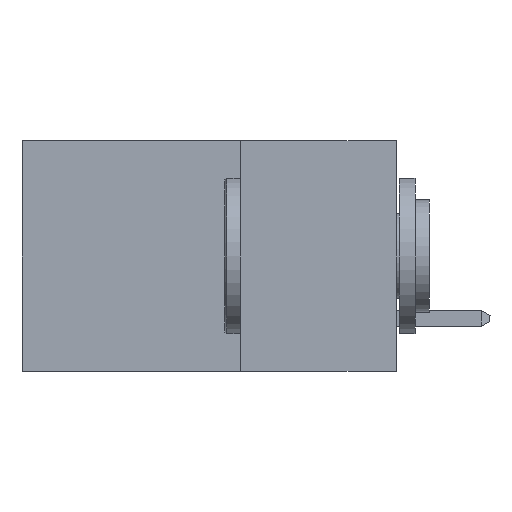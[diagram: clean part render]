
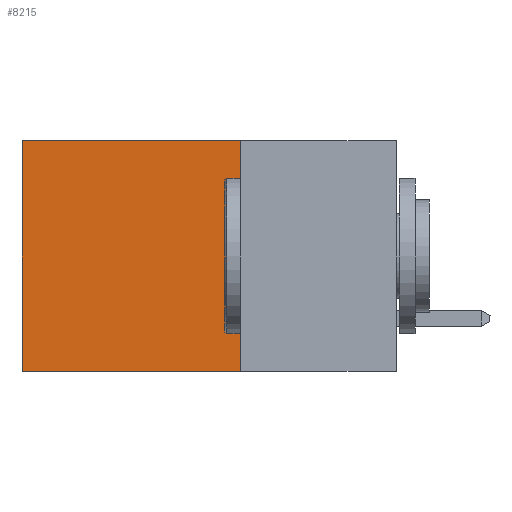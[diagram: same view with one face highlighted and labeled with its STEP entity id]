
A CAD part, left-side view. The second image highlights one B-rep face of the part: STEP entity #8215.
In plain terms, the highlighted planar face has unit normal (-1, 0, 0).
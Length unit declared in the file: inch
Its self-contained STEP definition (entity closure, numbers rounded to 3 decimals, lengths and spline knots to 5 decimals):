
#244 = VECTOR ( 'NONE', #9530, 39.37008 ) ;
#366 = VECTOR ( 'NONE', #10708, 39.37008 ) ;
#685 = VERTEX_POINT ( 'NONE', #2486 ) ;
#753 = EDGE_CURVE ( 'NONE', #7924, #6056, #8800, .T. ) ;
#1277 = EDGE_LOOP ( 'NONE', ( #5672, #1853, #2926, #5214 ) ) ;
#1853 = ORIENTED_EDGE ( 'NONE', *, *, #2600, .F. ) ;
#2177 = CARTESIAN_POINT ( 'NONE',  ( 0.2615, 0.25, -0.37 ) ) ;
#2486 = CARTESIAN_POINT ( 'NONE',  ( 0.2615, 0.6, -0.37 ) ) ;
#2600 = EDGE_CURVE ( 'NONE', #6056, #685, #5330, .T. ) ;
#2926 = ORIENTED_EDGE ( 'NONE', *, *, #753, .F. ) ;
#3370 = CARTESIAN_POINT ( 'NONE',  ( 0.2615, 0.25, -0.37 ) ) ;
#3420 = DIRECTION ( 'NONE',  ( 0., 0., -1. ) ) ;
#4081 = LINE ( 'NONE', #4215, #244 ) ;
#4215 = CARTESIAN_POINT ( 'NONE',  ( 0.2615, 0.6, -0.37 ) ) ;
#4459 = VERTEX_POINT ( 'NONE', #9785 ) ;
#5214 = ORIENTED_EDGE ( 'NONE', *, *, #10339, .T. ) ;
#5330 = LINE ( 'NONE', #9862, #366 ) ;
#5629 = EDGE_CURVE ( 'NONE', #4459, #685, #4081, .T. ) ;
#5672 = ORIENTED_EDGE ( 'NONE', *, *, #5629, .T. ) ;
#5827 = AXIS2_PLACEMENT_3D ( 'NONE', #3370, #8701, #7098 ) ;
#6056 = VERTEX_POINT ( 'NONE', #2177 ) ;
#7023 = CARTESIAN_POINT ( 'NONE',  ( 0.2615, 0.25, -0.37 ) ) ;
#7098 = DIRECTION ( 'NONE',  ( 0., 0., -1. ) ) ;
#7491 = LINE ( 'NONE', #9246, #8368 ) ;
#7924 = VERTEX_POINT ( 'NONE', #10249 ) ;
#8215 = ADVANCED_FACE ( 'NONE', ( #11293 ), #9685, .F. ) ;
#8368 = VECTOR ( 'NONE', #11036, 39.37008 ) ;
#8701 = DIRECTION ( 'NONE',  ( 1., 0., 0. ) ) ;
#8800 = LINE ( 'NONE', #7023, #10957 ) ;
#9246 = CARTESIAN_POINT ( 'NONE',  ( 0.2615, 0.25, 0. ) ) ;
#9530 = DIRECTION ( 'NONE',  ( 0., 0., -1. ) ) ;
#9685 = PLANE ( 'NONE',  #5827 ) ;
#9785 = CARTESIAN_POINT ( 'NONE',  ( 0.2615, 0.6, 0. ) ) ;
#9862 = CARTESIAN_POINT ( 'NONE',  ( 0.2615, 0.25, -0.37 ) ) ;
#10249 = CARTESIAN_POINT ( 'NONE',  ( 0.2615, 0.25, 0. ) ) ;
#10339 = EDGE_CURVE ( 'NONE', #7924, #4459, #7491, .T. ) ;
#10708 = DIRECTION ( 'NONE',  ( 0., 1., 0. ) ) ;
#10957 = VECTOR ( 'NONE', #3420, 39.37008 ) ;
#11036 = DIRECTION ( 'NONE',  ( 0., 1., 0. ) ) ;
#11293 = FACE_OUTER_BOUND ( 'NONE', #1277, .T. ) ;
